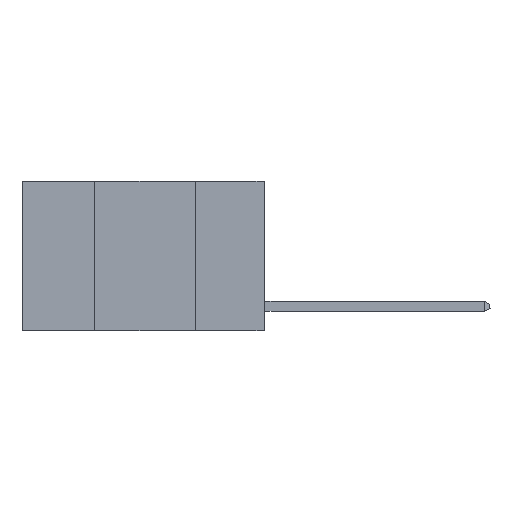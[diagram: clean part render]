
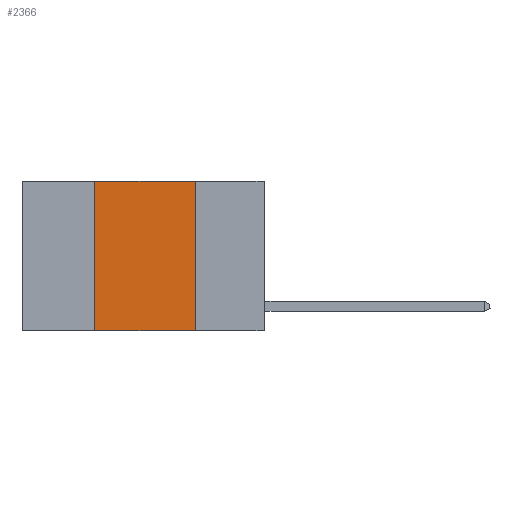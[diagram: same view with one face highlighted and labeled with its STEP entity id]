
A CAD part, left-side view. The second image highlights one B-rep face of the part: STEP entity #2366.
In plain terms, the highlighted planar face has unit normal (-1, 0, 0).
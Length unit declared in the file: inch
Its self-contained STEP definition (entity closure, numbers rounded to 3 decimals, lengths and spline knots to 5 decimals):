
#30 = VECTOR ( 'NONE', #8698, 39.37008 ) ;
#43 = EDGE_CURVE ( 'NONE', #5155, #3418, #7401, .T. ) ;
#98 = AXIS2_PLACEMENT_3D ( 'NONE', #2741, #7511, #8077 ) ;
#244 = CARTESIAN_POINT ( 'NONE',  ( 0., 0.6, 0. ) ) ;
#678 = ORIENTED_EDGE ( 'NONE', *, *, #1997, .F. ) ;
#959 = DIRECTION ( 'NONE',  ( 0., 0., -1. ) ) ;
#985 = CARTESIAN_POINT ( 'NONE',  ( 0., 0.42, 0. ) ) ;
#1424 = LINE ( 'NONE', #3285, #3221 ) ;
#1492 = ORIENTED_EDGE ( 'NONE', *, *, #43, .F. ) ;
#1691 = LINE ( 'NONE', #5007, #5415 ) ;
#1997 = EDGE_CURVE ( 'NONE', #3478, #8184, #1691, .T. ) ;
#2366 = ADVANCED_FACE ( 'NONE', ( #5411 ), #4831, .F. ) ;
#2396 = DIRECTION ( 'NONE',  ( 0., -1., 0. ) ) ;
#2663 = ORIENTED_EDGE ( 'NONE', *, *, #4709, .F. ) ;
#2741 = CARTESIAN_POINT ( 'NONE',  ( 0., 0.6, 0. ) ) ;
#2854 = ORIENTED_EDGE ( 'NONE', *, *, #6548, .T. ) ;
#3102 = CARTESIAN_POINT ( 'NONE',  ( 0., 0.17, -0.37 ) ) ;
#3221 = VECTOR ( 'NONE', #3968, 39.37008 ) ;
#3285 = CARTESIAN_POINT ( 'NONE',  ( 0., 0.6, -0.37 ) ) ;
#3418 = VERTEX_POINT ( 'NONE', #985 ) ;
#3478 = VERTEX_POINT ( 'NONE', #6866 ) ;
#3968 = DIRECTION ( 'NONE',  ( 0., -1., 0. ) ) ;
#4339 = EDGE_LOOP ( 'NONE', ( #678, #2663, #1492, #2854 ) ) ;
#4365 = LINE ( 'NONE', #244, #5045 ) ;
#4709 = EDGE_CURVE ( 'NONE', #3418, #3478, #4365, .T. ) ;
#4831 = PLANE ( 'NONE',  #98 ) ;
#5007 = CARTESIAN_POINT ( 'NONE',  ( 0., 0.17, 0. ) ) ;
#5045 = VECTOR ( 'NONE', #2396, 39.37008 ) ;
#5155 = VERTEX_POINT ( 'NONE', #5778 ) ;
#5411 = FACE_OUTER_BOUND ( 'NONE', #4339, .T. ) ;
#5415 = VECTOR ( 'NONE', #959, 39.37008 ) ;
#5778 = CARTESIAN_POINT ( 'NONE',  ( 0., 0.42, -0.37 ) ) ;
#5994 = CARTESIAN_POINT ( 'NONE',  ( 0., 0.42, 0. ) ) ;
#6548 = EDGE_CURVE ( 'NONE', #5155, #8184, #1424, .T. ) ;
#6866 = CARTESIAN_POINT ( 'NONE',  ( 0., 0.17, 0. ) ) ;
#7401 = LINE ( 'NONE', #5994, #30 ) ;
#7511 = DIRECTION ( 'NONE',  ( 1., 0., 0. ) ) ;
#8077 = DIRECTION ( 'NONE',  ( 0., 0., -1. ) ) ;
#8184 = VERTEX_POINT ( 'NONE', #3102 ) ;
#8698 = DIRECTION ( 'NONE',  ( 0., 0., 1. ) ) ;
